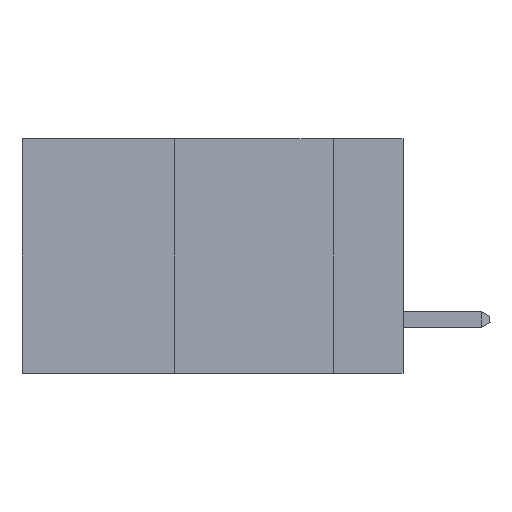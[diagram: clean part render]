
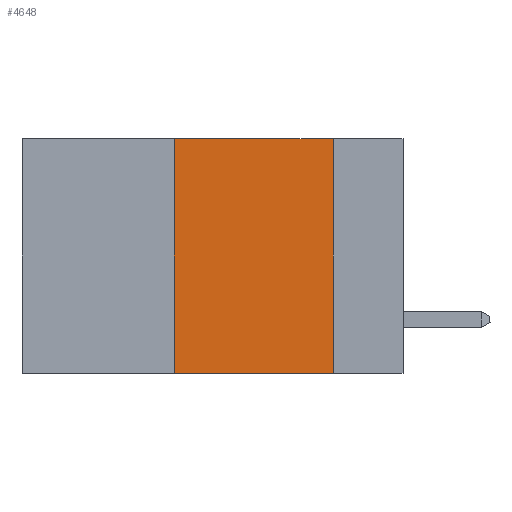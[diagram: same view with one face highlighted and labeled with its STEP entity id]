
A CAD part, left-side view. The second image highlights one B-rep face of the part: STEP entity #4648.
In plain terms, the highlighted planar face has unit normal (-1, 0, 0).
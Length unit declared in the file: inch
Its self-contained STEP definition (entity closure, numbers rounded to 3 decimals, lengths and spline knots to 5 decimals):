
#154 = VECTOR ( 'NONE', #2988, 39.37008 ) ;
#651 = LINE ( 'NONE', #1411, #154 ) ;
#1041 = EDGE_CURVE ( 'NONE', #7863, #1743, #5773, .T. ) ;
#1141 = CARTESIAN_POINT ( 'NONE',  ( 0., 0.11, 0. ) ) ;
#1411 = CARTESIAN_POINT ( 'NONE',  ( 0., 0.36, 0. ) ) ;
#1743 = VERTEX_POINT ( 'NONE', #17439 ) ;
#1829 = CARTESIAN_POINT ( 'NONE',  ( 0., 0.36, 0. ) ) ;
#2386 = VECTOR ( 'NONE', #12272, 39.37008 ) ;
#2716 = CARTESIAN_POINT ( 'NONE',  ( 0., 0.6, -0.37 ) ) ;
#2988 = DIRECTION ( 'NONE',  ( 0., 0., 1. ) ) ;
#3039 = EDGE_CURVE ( 'NONE', #11584, #7863, #13626, .T. ) ;
#3831 = VECTOR ( 'NONE', #12680, 39.37008 ) ;
#4359 = ORIENTED_EDGE ( 'NONE', *, *, #11394, .F. ) ;
#4648 = ADVANCED_FACE ( 'NONE', ( #9211 ), #6910, .F. ) ;
#4991 = EDGE_LOOP ( 'NONE', ( #18367, #18976, #4359, #15050 ) ) ;
#5773 = LINE ( 'NONE', #17808, #3831 ) ;
#6701 = AXIS2_PLACEMENT_3D ( 'NONE', #8425, #16559, #8774 ) ;
#6910 = PLANE ( 'NONE',  #6701 ) ;
#7863 = VERTEX_POINT ( 'NONE', #1141 ) ;
#8172 = CARTESIAN_POINT ( 'NONE',  ( 0., 0.36, -0.37 ) ) ;
#8202 = LINE ( 'NONE', #2716, #2386 ) ;
#8425 = CARTESIAN_POINT ( 'NONE',  ( 0., 0.6, 0. ) ) ;
#8437 = EDGE_CURVE ( 'NONE', #11079, #1743, #8202, .T. ) ;
#8513 = DIRECTION ( 'NONE',  ( 0., -1., 0. ) ) ;
#8774 = DIRECTION ( 'NONE',  ( 0., 0., -1. ) ) ;
#9211 = FACE_OUTER_BOUND ( 'NONE', #4991, .T. ) ;
#11079 = VERTEX_POINT ( 'NONE', #8172 ) ;
#11394 = EDGE_CURVE ( 'NONE', #11079, #11584, #651, .T. ) ;
#11584 = VERTEX_POINT ( 'NONE', #1829 ) ;
#12272 = DIRECTION ( 'NONE',  ( 0., -1., 0. ) ) ;
#12680 = DIRECTION ( 'NONE',  ( 0., 0., -1. ) ) ;
#13376 = VECTOR ( 'NONE', #8513, 39.37008 ) ;
#13626 = LINE ( 'NONE', #17804, #13376 ) ;
#15050 = ORIENTED_EDGE ( 'NONE', *, *, #8437, .T. ) ;
#16559 = DIRECTION ( 'NONE',  ( 1., 0., 0. ) ) ;
#17439 = CARTESIAN_POINT ( 'NONE',  ( 0., 0.11, -0.37 ) ) ;
#17804 = CARTESIAN_POINT ( 'NONE',  ( 0., 0.6, 0. ) ) ;
#17808 = CARTESIAN_POINT ( 'NONE',  ( 0., 0.11, 0. ) ) ;
#18367 = ORIENTED_EDGE ( 'NONE', *, *, #1041, .F. ) ;
#18976 = ORIENTED_EDGE ( 'NONE', *, *, #3039, .F. ) ;
